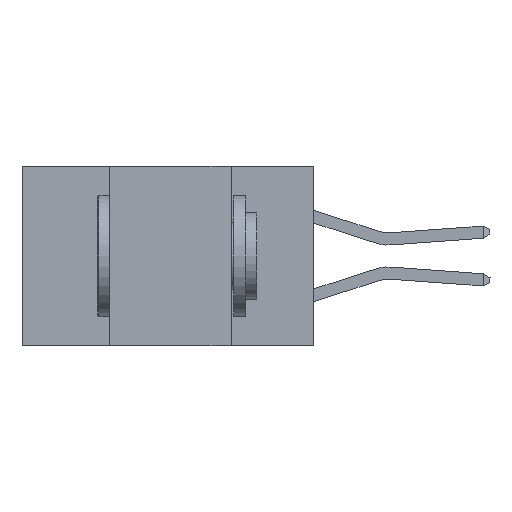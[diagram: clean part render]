
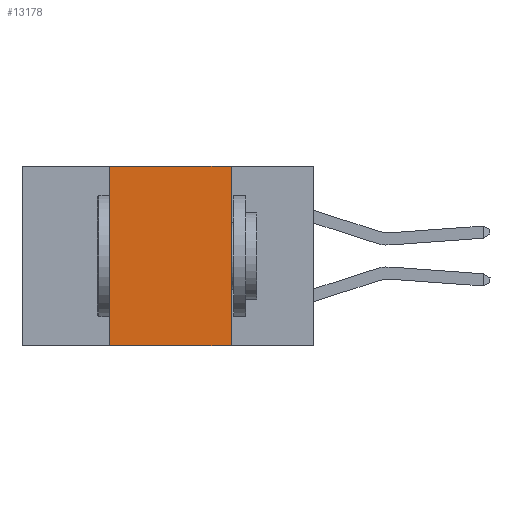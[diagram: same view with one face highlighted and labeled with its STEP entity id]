
A CAD part, left-side view. The second image highlights one B-rep face of the part: STEP entity #13178.
In plain terms, the highlighted planar face has unit normal (-1, 0, 0).
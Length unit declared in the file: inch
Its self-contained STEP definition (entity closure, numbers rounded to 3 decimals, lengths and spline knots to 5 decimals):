
#39 = CARTESIAN_POINT ( 'NONE',  ( 0., 0.6, 0. ) ) ;
#778 = LINE ( 'NONE', #13165, #13790 ) ;
#824 = VECTOR ( 'NONE', #2148, 39.37008 ) ;
#1220 = CARTESIAN_POINT ( 'NONE',  ( 0., 0.42, -0.37 ) ) ;
#2010 = EDGE_CURVE ( 'NONE', #6311, #4417, #6134, .T. ) ;
#2148 = DIRECTION ( 'NONE',  ( 0., -1., 0. ) ) ;
#2611 = CARTESIAN_POINT ( 'NONE',  ( 0., 0.42, 0. ) ) ;
#2788 = CARTESIAN_POINT ( 'NONE',  ( 0., 0.17, -0.37 ) ) ;
#2874 = ORIENTED_EDGE ( 'NONE', *, *, #5232, .F. ) ;
#3034 = EDGE_LOOP ( 'NONE', ( #9290, #11611, #2874, #10076 ) ) ;
#3534 = DIRECTION ( 'NONE',  ( 0., 0., -1. ) ) ;
#3796 = LINE ( 'NONE', #39, #824 ) ;
#4417 = VERTEX_POINT ( 'NONE', #2788 ) ;
#4648 = EDGE_CURVE ( 'NONE', #12549, #4417, #14233, .T. ) ;
#4901 = CARTESIAN_POINT ( 'NONE',  ( 0., 0.6, 0. ) ) ;
#5232 = EDGE_CURVE ( 'NONE', #12549, #13298, #778, .T. ) ;
#5247 = CARTESIAN_POINT ( 'NONE',  ( 0., 0.6, -0.37 ) ) ;
#6134 = LINE ( 'NONE', #10153, #12217 ) ;
#6146 = CARTESIAN_POINT ( 'NONE',  ( 0., 0.17, 0. ) ) ;
#6311 = VERTEX_POINT ( 'NONE', #6146 ) ;
#9196 = EDGE_CURVE ( 'NONE', #13298, #6311, #3796, .T. ) ;
#9290 = ORIENTED_EDGE ( 'NONE', *, *, #2010, .F. ) ;
#9514 = FACE_OUTER_BOUND ( 'NONE', #3034, .T. ) ;
#9882 = DIRECTION ( 'NONE',  ( 0., 0., 1. ) ) ;
#9913 = AXIS2_PLACEMENT_3D ( 'NONE', #4901, #11591, #11682 ) ;
#10076 = ORIENTED_EDGE ( 'NONE', *, *, #4648, .T. ) ;
#10153 = CARTESIAN_POINT ( 'NONE',  ( 0., 0.17, 0. ) ) ;
#11591 = DIRECTION ( 'NONE',  ( 1., 0., 0. ) ) ;
#11611 = ORIENTED_EDGE ( 'NONE', *, *, #9196, .F. ) ;
#11682 = DIRECTION ( 'NONE',  ( 0., 0., -1. ) ) ;
#12217 = VECTOR ( 'NONE', #3534, 39.37008 ) ;
#12549 = VERTEX_POINT ( 'NONE', #1220 ) ;
#13001 = DIRECTION ( 'NONE',  ( 0., -1., 0. ) ) ;
#13165 = CARTESIAN_POINT ( 'NONE',  ( 0., 0.42, 0. ) ) ;
#13178 = ADVANCED_FACE ( 'NONE', ( #9514 ), #13726, .F. ) ;
#13298 = VERTEX_POINT ( 'NONE', #2611 ) ;
#13726 = PLANE ( 'NONE',  #9913 ) ;
#13790 = VECTOR ( 'NONE', #9882, 39.37008 ) ;
#13873 = VECTOR ( 'NONE', #13001, 39.37008 ) ;
#14233 = LINE ( 'NONE', #5247, #13873 ) ;
